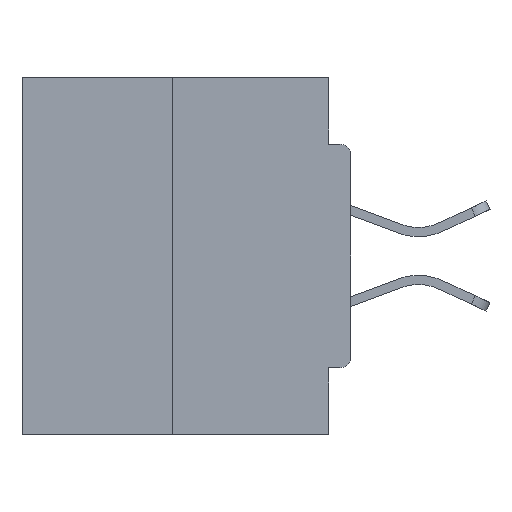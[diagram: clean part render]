
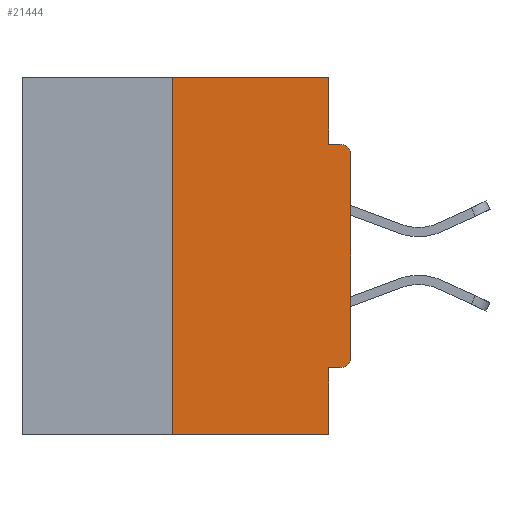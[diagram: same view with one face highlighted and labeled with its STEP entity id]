
A CAD part, left-side view. The second image highlights one B-rep face of the part: STEP entity #21444.
In plain terms, the highlighted planar face has unit normal (-1, 0, 0).
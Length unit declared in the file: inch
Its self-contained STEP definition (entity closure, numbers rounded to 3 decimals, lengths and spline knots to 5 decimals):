
#227 = DIRECTION ( 'NONE',  ( 0., 0., 1. ) ) ;
#447 = CARTESIAN_POINT ( 'NONE',  ( 0., 0.25, -0.5 ) ) ;
#1417 = DIRECTION ( 'NONE',  ( 0., 0., -1. ) ) ;
#1510 = VERTEX_POINT ( 'NONE', #19347 ) ;
#1826 = CIRCLE ( 'NONE', #5874, 0.015 ) ;
#2313 = EDGE_CURVE ( 'NONE', #16109, #8970, #13695, .T. ) ;
#3031 = CARTESIAN_POINT ( 'NONE',  ( 0., 0.015, -0.3915 ) ) ;
#3053 = CARTESIAN_POINT ( 'NONE',  ( 0., 0., 0. ) ) ;
#3977 = CIRCLE ( 'NONE', #13488, 0.015 ) ;
#4743 = VERTEX_POINT ( 'NONE', #15932 ) ;
#5545 = CARTESIAN_POINT ( 'NONE',  ( 0., 0.25, 0. ) ) ;
#5708 = CARTESIAN_POINT ( 'NONE',  ( 0., 0.031, -0.5 ) ) ;
#5874 = AXIS2_PLACEMENT_3D ( 'NONE', #3031, #28320, #11580 ) ;
#6477 = EDGE_CURVE ( 'NONE', #16109, #28921, #20425, .T. ) ;
#7533 = CARTESIAN_POINT ( 'NONE',  ( 0., 0., -0.1085 ) ) ;
#8023 = VECTOR ( 'NONE', #29524, 39.37008 ) ;
#8498 = DIRECTION ( 'NONE',  ( 0., -1., 0. ) ) ;
#8970 = VERTEX_POINT ( 'NONE', #19376 ) ;
#9363 = EDGE_CURVE ( 'NONE', #17166, #31221, #18434, .T. ) ;
#10769 = EDGE_CURVE ( 'NONE', #1510, #23004, #13322, .T. ) ;
#10864 = LINE ( 'NONE', #5708, #22212 ) ;
#10886 = CARTESIAN_POINT ( 'NONE',  ( 0., 0.031, 0. ) ) ;
#11004 = VECTOR ( 'NONE', #33413, 39.37008 ) ;
#11478 = VECTOR ( 'NONE', #227, 39.37008 ) ;
#11580 = DIRECTION ( 'NONE',  ( 0., 0., -1. ) ) ;
#11596 = CARTESIAN_POINT ( 'NONE',  ( 0., 0., -0.4065 ) ) ;
#12384 = EDGE_CURVE ( 'NONE', #31221, #23004, #3977, .T. ) ;
#13194 = LINE ( 'NONE', #11596, #19321 ) ;
#13230 = AXIS2_PLACEMENT_3D ( 'NONE', #18251, #35421, #1417 ) ;
#13232 = EDGE_CURVE ( 'NONE', #4743, #31222, #13194, .T. ) ;
#13322 = LINE ( 'NONE', #15676, #14222 ) ;
#13488 = AXIS2_PLACEMENT_3D ( 'NONE', #33141, #25453, #13915 ) ;
#13676 = DIRECTION ( 'NONE',  ( 0., 0., 1. ) ) ;
#13695 = LINE ( 'NONE', #5545, #30426 ) ;
#13915 = DIRECTION ( 'NONE',  ( 0., 0., -1. ) ) ;
#14222 = VECTOR ( 'NONE', #8498, 39.37008 ) ;
#14772 = VECTOR ( 'NONE', #30141, 39.37008 ) ;
#14968 = ORIENTED_EDGE ( 'NONE', *, *, #9363, .T. ) ;
#15676 = CARTESIAN_POINT ( 'NONE',  ( 0., 0., -0.0935 ) ) ;
#15760 = ORIENTED_EDGE ( 'NONE', *, *, #32672, .F. ) ;
#15816 = FACE_OUTER_BOUND ( 'NONE', #19135, .T. ) ;
#15932 = CARTESIAN_POINT ( 'NONE',  ( 0., 0.015, -0.4065 ) ) ;
#16109 = VERTEX_POINT ( 'NONE', #447 ) ;
#17019 = ORIENTED_EDGE ( 'NONE', *, *, #30494, .F. ) ;
#17166 = VERTEX_POINT ( 'NONE', #29489 ) ;
#17861 = CARTESIAN_POINT ( 'NONE',  ( 0., 0.031, -0.5 ) ) ;
#18251 = CARTESIAN_POINT ( 'NONE',  ( 0., 0.46, 0. ) ) ;
#18434 = LINE ( 'NONE', #3053, #11478 ) ;
#19135 = EDGE_LOOP ( 'NONE', ( #17019, #24020, #31930, #27205, #23780, #30492, #14968, #22000, #23015, #15760 ) ) ;
#19321 = VECTOR ( 'NONE', #22346, 39.37008 ) ;
#19328 = DIRECTION ( 'NONE',  ( 0., 0., -1. ) ) ;
#19347 = CARTESIAN_POINT ( 'NONE',  ( 0., 0.031, -0.0935 ) ) ;
#19376 = CARTESIAN_POINT ( 'NONE',  ( 0., 0.25, 0. ) ) ;
#20425 = LINE ( 'NONE', #35114, #14772 ) ;
#21444 = ADVANCED_FACE ( 'NONE', ( #15816 ), #29372, .F. ) ;
#22000 = ORIENTED_EDGE ( 'NONE', *, *, #12384, .T. ) ;
#22212 = VECTOR ( 'NONE', #19328, 39.37008 ) ;
#22346 = DIRECTION ( 'NONE',  ( 0., 1., 0. ) ) ;
#22495 = LINE ( 'NONE', #28929, #8023 ) ;
#23004 = VERTEX_POINT ( 'NONE', #32337 ) ;
#23015 = ORIENTED_EDGE ( 'NONE', *, *, #10769, .F. ) ;
#23780 = ORIENTED_EDGE ( 'NONE', *, *, #13232, .F. ) ;
#24020 = ORIENTED_EDGE ( 'NONE', *, *, #2313, .F. ) ;
#25453 = DIRECTION ( 'NONE',  ( -1., 0., 0. ) ) ;
#26339 = LINE ( 'NONE', #10886, #11004 ) ;
#27205 = ORIENTED_EDGE ( 'NONE', *, *, #34621, .F. ) ;
#28320 = DIRECTION ( 'NONE',  ( -1., 0., 0. ) ) ;
#28921 = VERTEX_POINT ( 'NONE', #17861 ) ;
#28929 = CARTESIAN_POINT ( 'NONE',  ( 0., 0.46, 0. ) ) ;
#29372 = PLANE ( 'NONE',  #13230 ) ;
#29489 = CARTESIAN_POINT ( 'NONE',  ( 0., 0., -0.3915 ) ) ;
#29524 = DIRECTION ( 'NONE',  ( 0., -1., 0. ) ) ;
#30072 = CARTESIAN_POINT ( 'NONE',  ( 0., 0.031, -0.4065 ) ) ;
#30141 = DIRECTION ( 'NONE',  ( 0., -1., 0. ) ) ;
#30262 = EDGE_CURVE ( 'NONE', #4743, #17166, #1826, .T. ) ;
#30426 = VECTOR ( 'NONE', #13676, 39.37008 ) ;
#30492 = ORIENTED_EDGE ( 'NONE', *, *, #30262, .T. ) ;
#30494 = EDGE_CURVE ( 'NONE', #8970, #32360, #22495, .T. ) ;
#31221 = VERTEX_POINT ( 'NONE', #7533 ) ;
#31222 = VERTEX_POINT ( 'NONE', #30072 ) ;
#31930 = ORIENTED_EDGE ( 'NONE', *, *, #6477, .T. ) ;
#32337 = CARTESIAN_POINT ( 'NONE',  ( 0., 0.015, -0.0935 ) ) ;
#32360 = VERTEX_POINT ( 'NONE', #34637 ) ;
#32672 = EDGE_CURVE ( 'NONE', #32360, #1510, #26339, .T. ) ;
#33141 = CARTESIAN_POINT ( 'NONE',  ( 0., 0.015, -0.1085 ) ) ;
#33413 = DIRECTION ( 'NONE',  ( 0., 0., -1. ) ) ;
#34621 = EDGE_CURVE ( 'NONE', #31222, #28921, #10864, .T. ) ;
#34637 = CARTESIAN_POINT ( 'NONE',  ( 0., 0.031, 0. ) ) ;
#35114 = CARTESIAN_POINT ( 'NONE',  ( 0., 0.46, -0.5 ) ) ;
#35421 = DIRECTION ( 'NONE',  ( 1., 0., 0. ) ) ;
